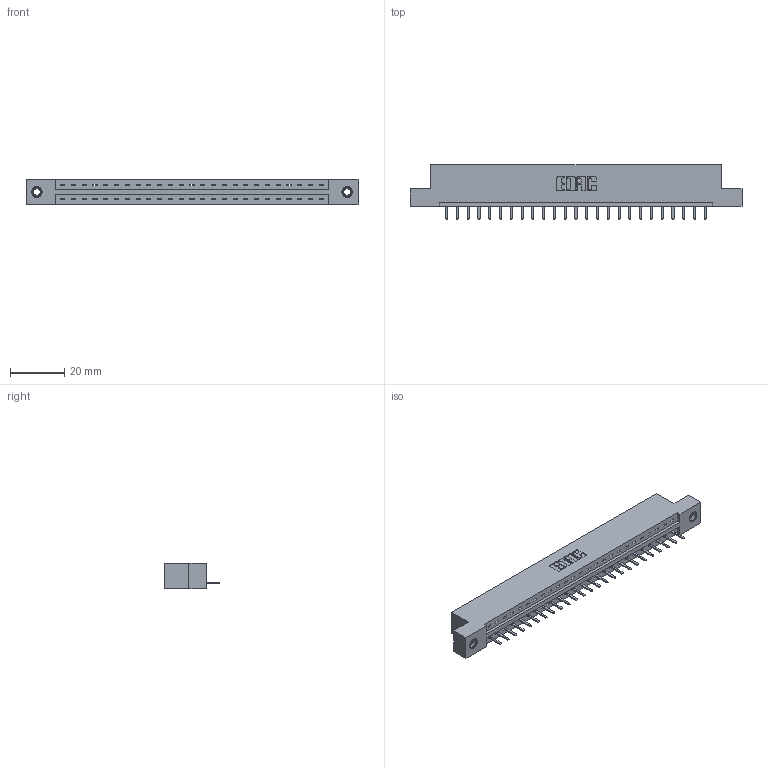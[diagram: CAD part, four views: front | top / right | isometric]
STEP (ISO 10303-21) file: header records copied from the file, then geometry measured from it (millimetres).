
FILE_DESCRIPTION (( 'STEP AP203' ), '1' );
FILE_NAME ('337-025-520-107.STEP', '2019-09-30T16:27:17', ( '' ), ( '' ), 'SwSTEP 2.0', 'SolidWorks 2016', '' );
FILE_SCHEMA (( 'CONFIG_CONTROL_DESIGN' ));
Length unit declared in the file: inch
Products named in the file (4): 337 Part_Flush Mounting Lugs - 0.156 Dia-TI; 345-292-001_345-293-120; 345-250-001_345-250-005-103; 337-025-520-107
Assembly tree (28 placements, depth 2):
  337-025-520-107
    337 Part_Flush Mounting Lugs - 0.156 Dia-TI
    345-292-001_345-293-120  x25
    345-250-001_345-250-005-103  x2
Bounding box: 122.07 x 20.02 x 9.4 mm (x, y, z)
Volume: 12389.2 mm3; surface area: 12490.3 mm2
Topology: 28 solids, 28 shells, 1824 faces, 5347 edges, 3490 vertices
Faces by surface type: plane 1302, cylinder 506, cone 12, torus 4
Entity records: 22082 total; most frequent: CARTESIAN_POINT 3836, ORIENTED_EDGE 3778, DIRECTION 3285, EDGE_CURVE 1889, VECTOR 1737, LINE 1737, VERTEX_POINT 1252, AXIS2_PLACEMENT_3D 774
